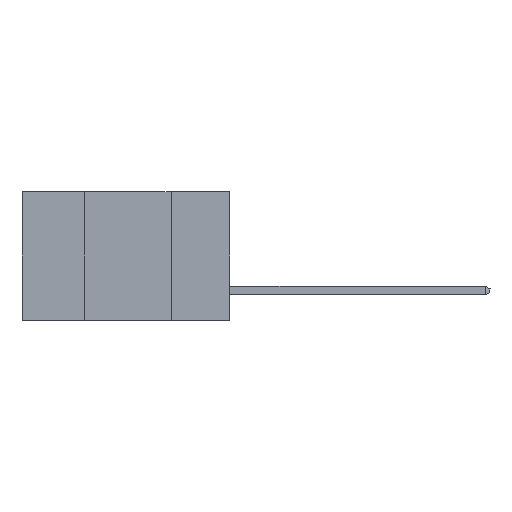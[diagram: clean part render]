
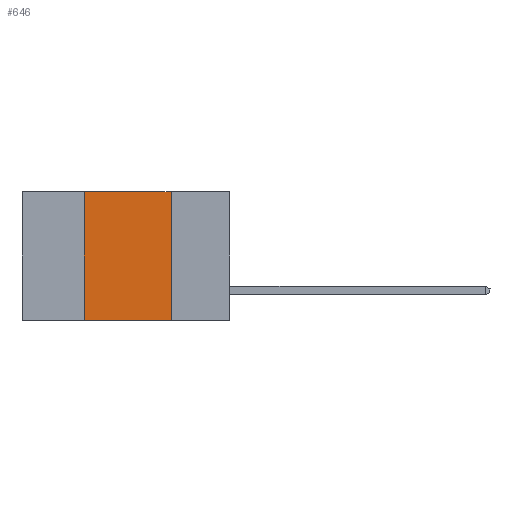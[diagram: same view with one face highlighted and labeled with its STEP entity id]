
A CAD part, left-side view. The second image highlights one B-rep face of the part: STEP entity #646.
In plain terms, the highlighted planar face has unit normal (-1, 0, 0).
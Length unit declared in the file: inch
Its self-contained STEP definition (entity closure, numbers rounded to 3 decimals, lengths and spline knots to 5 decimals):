
#153 = CARTESIAN_POINT ( 'NONE',  ( 0., 0.42, -0.37 ) ) ;
#263 = ORIENTED_EDGE ( 'NONE', *, *, #10101, .T. ) ;
#552 = VERTEX_POINT ( 'NONE', #4278 ) ;
#646 = ADVANCED_FACE ( 'NONE', ( #4389 ), #5330, .F. ) ;
#1821 = DIRECTION ( 'NONE',  ( 0., 0., -1. ) ) ;
#2145 = CARTESIAN_POINT ( 'NONE',  ( 0., 0.6, 0. ) ) ;
#2196 = EDGE_CURVE ( 'NONE', #552, #11849, #6800, .T. ) ;
#2530 = EDGE_LOOP ( 'NONE', ( #12066, #9145, #6203, #263 ) ) ;
#3049 = VERTEX_POINT ( 'NONE', #11268 ) ;
#3523 = LINE ( 'NONE', #4561, #5182 ) ;
#3596 = DIRECTION ( 'NONE',  ( 0., 0., 1. ) ) ;
#3782 = DIRECTION ( 'NONE',  ( 0., -1., 0. ) ) ;
#4278 = CARTESIAN_POINT ( 'NONE',  ( 0., 0.42, 0. ) ) ;
#4389 = FACE_OUTER_BOUND ( 'NONE', #2530, .T. ) ;
#4561 = CARTESIAN_POINT ( 'NONE',  ( 0., 0.6, -0.37 ) ) ;
#5182 = VECTOR ( 'NONE', #11902, 39.37008 ) ;
#5330 = PLANE ( 'NONE',  #7087 ) ;
#5369 = VECTOR ( 'NONE', #3596, 39.37008 ) ;
#6203 = ORIENTED_EDGE ( 'NONE', *, *, #9711, .F. ) ;
#6424 = CARTESIAN_POINT ( 'NONE',  ( 0., 0.6, 0. ) ) ;
#6659 = DIRECTION ( 'NONE',  ( 0., 0., -1. ) ) ;
#6800 = LINE ( 'NONE', #2145, #9536 ) ;
#7087 = AXIS2_PLACEMENT_3D ( 'NONE', #6424, #8153, #1821 ) ;
#7168 = LINE ( 'NONE', #9074, #5369 ) ;
#8153 = DIRECTION ( 'NONE',  ( 1., 0., 0. ) ) ;
#8447 = LINE ( 'NONE', #10353, #11480 ) ;
#9074 = CARTESIAN_POINT ( 'NONE',  ( 0., 0.42, -0.37 ) ) ;
#9145 = ORIENTED_EDGE ( 'NONE', *, *, #2196, .F. ) ;
#9536 = VECTOR ( 'NONE', #3782, 39.37008 ) ;
#9711 = EDGE_CURVE ( 'NONE', #11935, #552, #7168, .T. ) ;
#10101 = EDGE_CURVE ( 'NONE', #11935, #3049, #3523, .T. ) ;
#10353 = CARTESIAN_POINT ( 'NONE',  ( 0., 0.17, -0.37 ) ) ;
#11268 = CARTESIAN_POINT ( 'NONE',  ( 0., 0.17, -0.37 ) ) ;
#11480 = VECTOR ( 'NONE', #6659, 39.37008 ) ;
#11584 = EDGE_CURVE ( 'NONE', #11849, #3049, #8447, .T. ) ;
#11826 = CARTESIAN_POINT ( 'NONE',  ( 0., 0.17, 0. ) ) ;
#11849 = VERTEX_POINT ( 'NONE', #11826 ) ;
#11902 = DIRECTION ( 'NONE',  ( 0., -1., 0. ) ) ;
#11935 = VERTEX_POINT ( 'NONE', #153 ) ;
#12066 = ORIENTED_EDGE ( 'NONE', *, *, #11584, .F. ) ;
